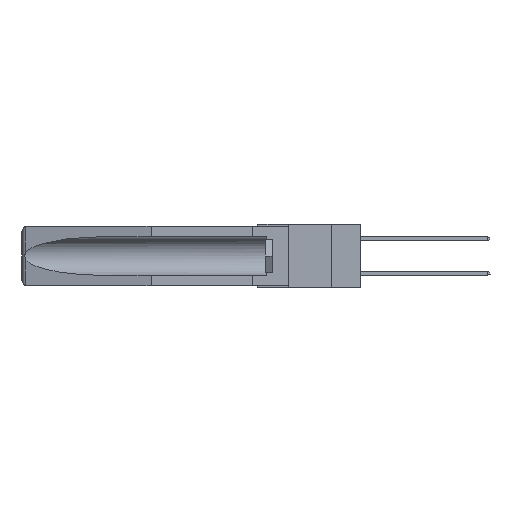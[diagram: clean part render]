
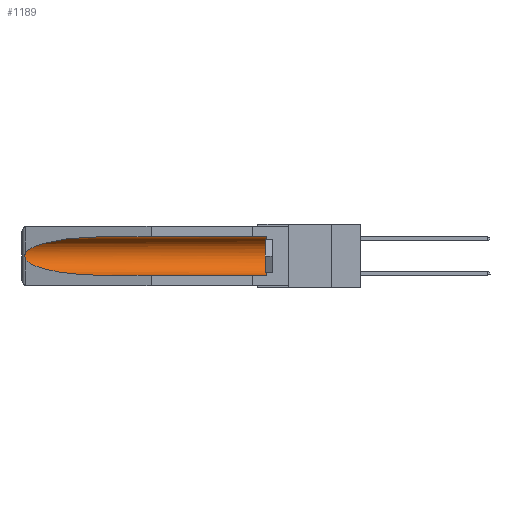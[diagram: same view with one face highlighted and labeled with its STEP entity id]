
A CAD part, left-side view. The second image highlights one B-rep face of the part: STEP entity #1189.
In plain terms, the highlighted cylindrical face has radius 2.857 mm (diameter 5.715 mm), a partial arc.
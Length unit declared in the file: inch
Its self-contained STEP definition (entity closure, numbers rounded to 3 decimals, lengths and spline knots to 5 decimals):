
#41 = VERTEX_POINT ( 'NONE', #12248 ) ;
#401 = CARTESIAN_POINT ( 'NONE',  ( 0.155, 1.07973, -0.284 ) ) ;
#534 = CARTESIAN_POINT ( 'NONE',  ( 0.155, 1.07973, -0.059 ) ) ;
#808 = CARTESIAN_POINT ( 'NONE',  ( 0.2675, 1.53308, -0.17534 ) ) ;
#857 = VERTEX_POINT ( 'NONE', #7769 ) ;
#1189 = ADVANCED_FACE ( 'NONE', ( #6660 ), #16032, .F. ) ;
#1405 = VERTEX_POINT ( 'NONE', #3911 ) ;
#1791 = ORIENTED_EDGE ( 'NONE', *, *, #3354, .T. ) ;
#1811 = ORIENTED_EDGE ( 'NONE', *, *, #7057, .T. ) ;
#2305 = ORIENTED_EDGE ( 'NONE', *, *, #7008, .F. ) ;
#2338 = CARTESIAN_POINT ( 'NONE',  ( 0.26537, 1.52718, -0.19328 ) ) ;
#3154 = ORIENTED_EDGE ( 'NONE', *, *, #4894, .T. ) ;
#3354 = EDGE_CURVE ( 'NONE', #1405, #18327, #18808, .T. ) ;
#3911 = CARTESIAN_POINT ( 'NONE',  ( 0.155, 0.126, -0.059 ) ) ;
#3975 = CARTESIAN_POINT ( 'NONE',  ( 0.26537, 1.52718, -0.14972 ) ) ;
#4894 = EDGE_CURVE ( 'NONE', #857, #1405, #7778, .T. ) ;
#5252 = EDGE_CURVE ( 'NONE', #18327, #6675, #9352, .T. ) ;
#5291 = CARTESIAN_POINT ( 'NONE',  ( 0.26654, 1.53092, -0.15636 ) ) ;
#5649 = DIRECTION ( 'NONE',  ( 0., 1., 0. ) ) ;
#5826 = VERTEX_POINT ( 'NONE', #6555 ) ;
#6003 = CARTESIAN_POINT ( 'NONE',  ( 0.155, -0.30754, -0.284 ) ) ;
#6377 = CARTESIAN_POINT ( 'NONE',  ( 0.155, 1.07973, -0.059 ) ) ;
#6555 = CARTESIAN_POINT ( 'NONE',  ( 0.155, 1.07973, -0.284 ) ) ;
#6583 = CARTESIAN_POINT ( 'NONE',  ( 0.21114, 1.30732, -0.059 ) ) ;
#6660 = FACE_OUTER_BOUND ( 'NONE', #11831, .T. ) ;
#6675 = VERTEX_POINT ( 'NONE', #18940 ) ;
#6927 = CARTESIAN_POINT ( 'NONE',  ( 0.26655, 1.53094, -0.18657 ) ) ;
#7008 = EDGE_CURVE ( 'NONE', #857, #5826, #10963, .T. ) ;
#7057 = EDGE_CURVE ( 'NONE', #41, #5826, #12821, .T. ) ;
#7544 = VECTOR ( 'NONE', #5649, 39.37008 ) ;
#7769 = CARTESIAN_POINT ( 'NONE',  ( 0.155, 0.126, -0.284 ) ) ;
#7778 = CIRCLE ( 'NONE', #9392, 0.1125 ) ;
#7809 = CARTESIAN_POINT ( 'NONE',  ( 0.26537, 1.52718, -0.14972 ) ) ;
#7898 = CARTESIAN_POINT ( 'NONE',  ( 0.21114, 1.30732, -0.284 ) ) ;
#7921 = DIRECTION ( 'NONE',  ( 0., 1., 0. ) ) ;
#8632 = ORIENTED_EDGE ( 'NONE', *, *, #5252, .T. ) ;
#9005 = DIRECTION ( 'NONE',  ( 0., 0., 1. ) ) ;
#9352 =( BOUNDED_CURVE ( )  B_SPLINE_CURVE ( 3, ( #534, #6583, #13715, #7809 ),
 .UNSPECIFIED., .F., .F. ) 
 B_SPLINE_CURVE_WITH_KNOTS ( ( 4, 4 ),
 ( 4.71239, 6.08839 ),
 .UNSPECIFIED. ) 
 CURVE ( )  GEOMETRIC_REPRESENTATION_ITEM ( )  RATIONAL_B_SPLINE_CURVE ( ( 1., 0.848, 0.848, 1. ) ) 
 REPRESENTATION_ITEM ( '' )  );
#9392 = AXIS2_PLACEMENT_3D ( 'NONE', #14512, #13156, #13408 ) ;
#9475 = CARTESIAN_POINT ( 'NONE',  ( 0.26537, 1.52718, -0.19328 ) ) ;
#9818 = CARTESIAN_POINT ( 'NONE',  ( 0.26597, 1.5296, -0.19026 ) ) ;
#10963 = LINE ( 'NONE', #6003, #14715 ) ;
#11831 = EDGE_LOOP ( 'NONE', ( #8632, #15398, #1811, #2305, #3154, #1791 ) ) ;
#11895 = EDGE_CURVE ( 'NONE', #6675, #41, #18351, .T. ) ;
#12248 = CARTESIAN_POINT ( 'NONE',  ( 0.26537, 1.52718, -0.19328 ) ) ;
#12292 = CARTESIAN_POINT ( 'NONE',  ( 0.25451, 1.48313, -0.24835 ) ) ;
#12762 = CARTESIAN_POINT ( 'NONE',  ( 0.26597, 1.52961, -0.15275 ) ) ;
#12821 =( BOUNDED_CURVE ( )  B_SPLINE_CURVE ( 3, ( #9475, #12292, #7898, #401 ),
 .UNSPECIFIED., .F., .F. ) 
 B_SPLINE_CURVE_WITH_KNOTS ( ( 4, 4 ),
 ( 0.1948, 1.5708 ),
 .UNSPECIFIED. ) 
 CURVE ( )  GEOMETRIC_REPRESENTATION_ITEM ( )  RATIONAL_B_SPLINE_CURVE ( ( 1., 0.848, 0.848, 1. ) ) 
 REPRESENTATION_ITEM ( '' )  );
#13156 = DIRECTION ( 'NONE',  ( 0., -1., 0. ) ) ;
#13408 = DIRECTION ( 'NONE',  ( 0., 0., 1. ) ) ;
#13715 = CARTESIAN_POINT ( 'NONE',  ( 0.25451, 1.48313, -0.09465 ) ) ;
#14458 = CARTESIAN_POINT ( 'NONE',  ( 0.2673, 1.5327, -0.16383 ) ) ;
#14512 = CARTESIAN_POINT ( 'NONE',  ( 0.155, 0.126, -0.1715 ) ) ;
#14695 = CARTESIAN_POINT ( 'NONE',  ( 0.155, -0.30754, -0.059 ) ) ;
#14715 = VECTOR ( 'NONE', #16661, 39.37008 ) ;
#15398 = ORIENTED_EDGE ( 'NONE', *, *, #11895, .T. ) ;
#16032 = CYLINDRICAL_SURFACE ( 'NONE', #16746, 0.1125 ) ;
#16661 = DIRECTION ( 'NONE',  ( 0., 1., 0. ) ) ;
#16746 = AXIS2_PLACEMENT_3D ( 'NONE', #18037, #7921, #9005 ) ;
#17260 = CARTESIAN_POINT ( 'NONE',  ( 0.2675, 1.53308, -0.16763 ) ) ;
#18037 = CARTESIAN_POINT ( 'NONE',  ( 0.155, -0.30754, -0.1715 ) ) ;
#18327 = VERTEX_POINT ( 'NONE', #6377 ) ;
#18351 = B_SPLINE_CURVE_WITH_KNOTS ( 'NONE', 3,
 ( #3975, #12762, #5291, #14458, #17260, #808, #18806, #6927, #9818, #2338 ),
 .UNSPECIFIED., .F., .F.,
 ( 4, 2, 2, 2, 4 ),
 ( 0., 0.00029, 0.00058, 0.00087, 0.00117 ),
 .UNSPECIFIED. ) ;
#18806 = CARTESIAN_POINT ( 'NONE',  ( 0.2673, 1.53269, -0.17917 ) ) ;
#18808 = LINE ( 'NONE', #14695, #7544 ) ;
#18940 = CARTESIAN_POINT ( 'NONE',  ( 0.26537, 1.52718, -0.14972 ) ) ;
